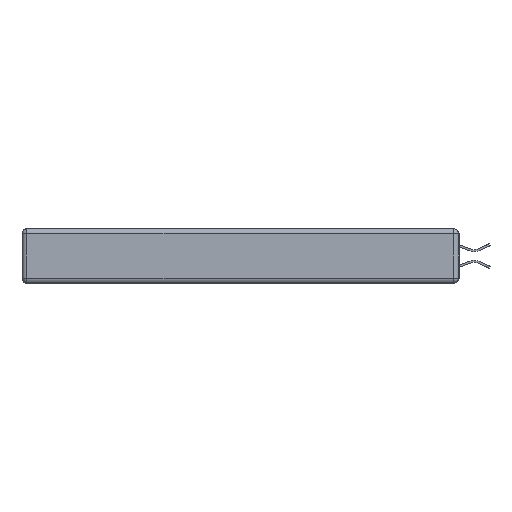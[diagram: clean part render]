
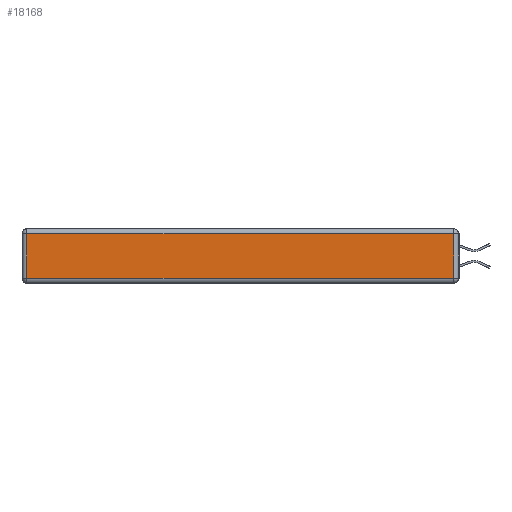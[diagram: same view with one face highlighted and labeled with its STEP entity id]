
A CAD part, left-side view. The second image highlights one B-rep face of the part: STEP entity #18168.
In plain terms, the highlighted planar face has unit normal (-1, 0, 0).
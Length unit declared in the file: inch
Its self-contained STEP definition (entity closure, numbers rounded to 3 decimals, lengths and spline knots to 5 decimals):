
#1975 = CARTESIAN_POINT ( 'NONE',  ( 0., 0.03, -0.343 ) ) ;
#2050 = EDGE_CURVE ( 'NONE', #17540, #10641, #25166, .T. ) ;
#2189 = DIRECTION ( 'NONE',  ( 0., 1., 0. ) ) ;
#2515 = DIRECTION ( 'NONE',  ( 0., 0., 1. ) ) ;
#4627 = CARTESIAN_POINT ( 'NONE',  ( 0., 0., -0.313 ) ) ;
#9090 = AXIS2_PLACEMENT_3D ( 'NONE', #32399, #9569, #17046 ) ;
#9569 = DIRECTION ( 'NONE',  ( -1., 0., 0. ) ) ;
#10092 = EDGE_LOOP ( 'NONE', ( #30794, #12535, #16168, #24127 ) ) ;
#10641 = VERTEX_POINT ( 'NONE', #10903 ) ;
#10903 = CARTESIAN_POINT ( 'NONE',  ( 0., 0.03, -0.313 ) ) ;
#12076 = VERTEX_POINT ( 'NONE', #28534 ) ;
#12535 = ORIENTED_EDGE ( 'NONE', *, *, #18821, .T. ) ;
#14102 = VERTEX_POINT ( 'NONE', #20413 ) ;
#15936 = VECTOR ( 'NONE', #2515, 39.37008 ) ;
#16168 = ORIENTED_EDGE ( 'NONE', *, *, #16221, .T. ) ;
#16221 = EDGE_CURVE ( 'NONE', #14102, #12076, #33075, .T. ) ;
#16242 = VECTOR ( 'NONE', #2189, 39.37008 ) ;
#16973 = VECTOR ( 'NONE', #23061, 39.37008 ) ;
#17046 = DIRECTION ( 'NONE',  ( 0., 0., 1. ) ) ;
#17540 = VERTEX_POINT ( 'NONE', #30156 ) ;
#18168 = ADVANCED_FACE ( 'NONE', ( #20816 ), #19331, .T. ) ;
#18392 = VECTOR ( 'NONE', #25371, 39.37008 ) ;
#18821 = EDGE_CURVE ( 'NONE', #10641, #14102, #20790, .T. ) ;
#19331 = PLANE ( 'NONE',  #9090 ) ;
#19471 = LINE ( 'NONE', #20398, #16973 ) ;
#20398 = CARTESIAN_POINT ( 'NONE',  ( 0., 2.72, -0.343 ) ) ;
#20413 = CARTESIAN_POINT ( 'NONE',  ( 0., 0.03, -0.03 ) ) ;
#20790 = LINE ( 'NONE', #1975, #15936 ) ;
#20816 = FACE_OUTER_BOUND ( 'NONE', #10092, .T. ) ;
#23061 = DIRECTION ( 'NONE',  ( 0., 0., -1. ) ) ;
#24127 = ORIENTED_EDGE ( 'NONE', *, *, #25326, .T. ) ;
#25166 = LINE ( 'NONE', #4627, #18392 ) ;
#25326 = EDGE_CURVE ( 'NONE', #12076, #17540, #19471, .T. ) ;
#25371 = DIRECTION ( 'NONE',  ( 0., -1., 0. ) ) ;
#25604 = CARTESIAN_POINT ( 'NONE',  ( 0., 2.75, -0.03 ) ) ;
#28534 = CARTESIAN_POINT ( 'NONE',  ( 0., 2.72, -0.03 ) ) ;
#30156 = CARTESIAN_POINT ( 'NONE',  ( 0., 2.72, -0.313 ) ) ;
#30794 = ORIENTED_EDGE ( 'NONE', *, *, #2050, .T. ) ;
#32399 = CARTESIAN_POINT ( 'NONE',  ( 0., 0., -0.343 ) ) ;
#33075 = LINE ( 'NONE', #25604, #16242 ) ;
